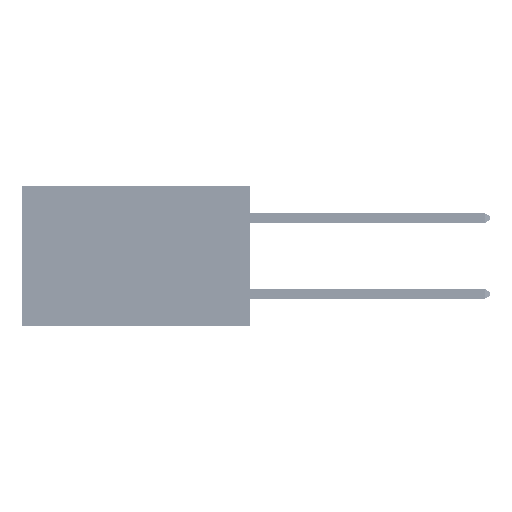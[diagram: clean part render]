
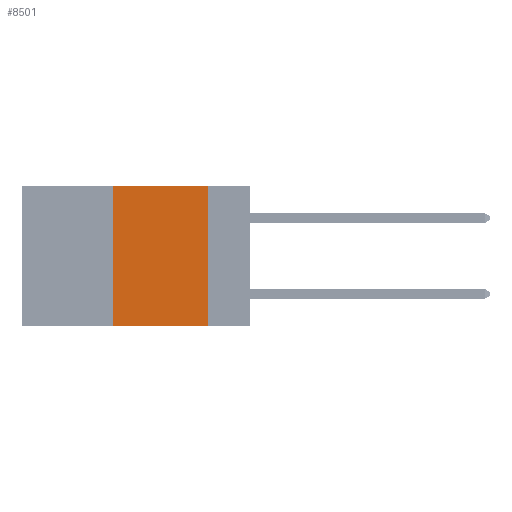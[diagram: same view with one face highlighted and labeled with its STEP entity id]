
A CAD part, left-side view. The second image highlights one B-rep face of the part: STEP entity #8501.
In plain terms, the highlighted planar face has unit normal (-1, 0, 0).
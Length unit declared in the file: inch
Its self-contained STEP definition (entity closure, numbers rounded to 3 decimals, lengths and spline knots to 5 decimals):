
#1075 = EDGE_CURVE ( 'NONE', #12423, #2053, #29358, .T. ) ;
#1637 = DIRECTION ( 'NONE',  ( 1., 0., 0. ) ) ;
#2053 = VERTEX_POINT ( 'NONE', #44265 ) ;
#2106 = FACE_OUTER_BOUND ( 'NONE', #26353, .T. ) ;
#2811 = VECTOR ( 'NONE', #3330, 39.37008 ) ;
#3330 = DIRECTION ( 'NONE',  ( 0., 0., -1. ) ) ;
#6609 = AXIS2_PLACEMENT_3D ( 'NONE', #34856, #1637, #20506 ) ;
#8501 = ADVANCED_FACE ( 'NONE', ( #2106 ), #27439, .F. ) ;
#9087 = DIRECTION ( 'NONE',  ( 0., 0., 1. ) ) ;
#9420 = EDGE_CURVE ( 'NONE', #41583, #12423, #45914, .T. ) ;
#10212 = EDGE_CURVE ( 'NONE', #19240, #2053, #22546, .T. ) ;
#10845 = DIRECTION ( 'NONE',  ( 0., -1., 0. ) ) ;
#11139 = ORIENTED_EDGE ( 'NONE', *, *, #13506, .F. ) ;
#12423 = VERTEX_POINT ( 'NONE', #21488 ) ;
#13013 = ORIENTED_EDGE ( 'NONE', *, *, #1075, .F. ) ;
#13171 = CARTESIAN_POINT ( 'NONE',  ( 0., 0.6, 0. ) ) ;
#13506 = EDGE_CURVE ( 'NONE', #19240, #41583, #26779, .T. ) ;
#14241 = ORIENTED_EDGE ( 'NONE', *, *, #10212, .T. ) ;
#15957 = VECTOR ( 'NONE', #9087, 39.37008 ) ;
#19240 = VERTEX_POINT ( 'NONE', #32310 ) ;
#20506 = DIRECTION ( 'NONE',  ( 0., 0., -1. ) ) ;
#21488 = CARTESIAN_POINT ( 'NONE',  ( 0., 0.11, 0. ) ) ;
#22310 = CARTESIAN_POINT ( 'NONE',  ( 0., 0.6, -0.37 ) ) ;
#22546 = LINE ( 'NONE', #22310, #37985 ) ;
#25739 = VECTOR ( 'NONE', #27741, 39.37008 ) ;
#26353 = EDGE_LOOP ( 'NONE', ( #13013, #27119, #11139, #14241 ) ) ;
#26779 = LINE ( 'NONE', #27253, #15957 ) ;
#27119 = ORIENTED_EDGE ( 'NONE', *, *, #9420, .F. ) ;
#27253 = CARTESIAN_POINT ( 'NONE',  ( 0., 0.36, 0. ) ) ;
#27439 = PLANE ( 'NONE',  #6609 ) ;
#27741 = DIRECTION ( 'NONE',  ( 0., -1., 0. ) ) ;
#28873 = CARTESIAN_POINT ( 'NONE',  ( 0., 0.11, 0. ) ) ;
#29358 = LINE ( 'NONE', #28873, #2811 ) ;
#32310 = CARTESIAN_POINT ( 'NONE',  ( 0., 0.36, -0.37 ) ) ;
#34856 = CARTESIAN_POINT ( 'NONE',  ( 0., 0.6, 0. ) ) ;
#37985 = VECTOR ( 'NONE', #10845, 39.37008 ) ;
#41583 = VERTEX_POINT ( 'NONE', #44278 ) ;
#44265 = CARTESIAN_POINT ( 'NONE',  ( 0., 0.11, -0.37 ) ) ;
#44278 = CARTESIAN_POINT ( 'NONE',  ( 0., 0.36, 0. ) ) ;
#45914 = LINE ( 'NONE', #13171, #25739 ) ;
